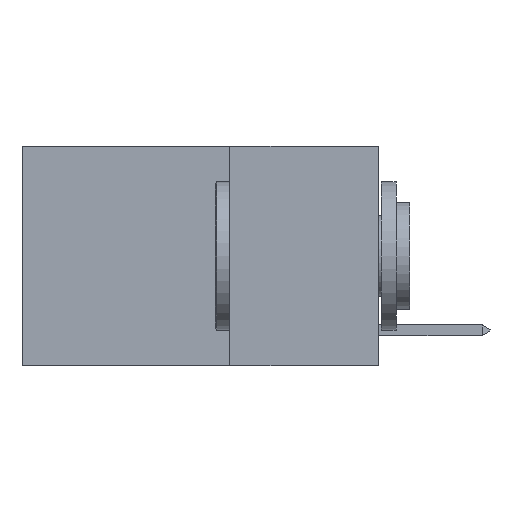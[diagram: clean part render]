
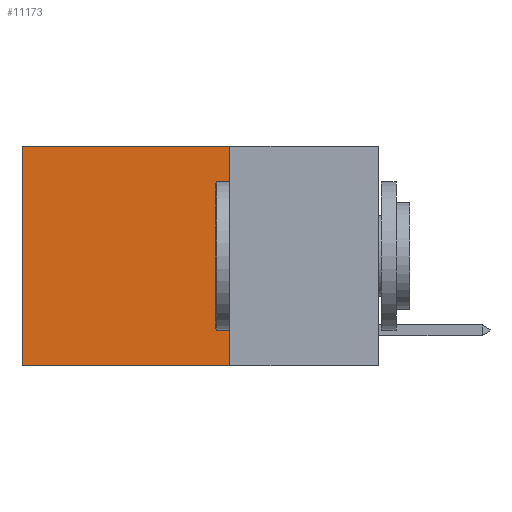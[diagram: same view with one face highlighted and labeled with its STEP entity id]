
A CAD part, left-side view. The second image highlights one B-rep face of the part: STEP entity #11173.
In plain terms, the highlighted planar face has unit normal (-1, 0, 0).
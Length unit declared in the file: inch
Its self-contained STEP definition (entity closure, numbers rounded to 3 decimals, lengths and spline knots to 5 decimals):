
#128 = CARTESIAN_POINT ( 'NONE',  ( 0.2625, 0.25, 0. ) ) ;
#1130 = VERTEX_POINT ( 'NONE', #2008 ) ;
#1347 = CARTESIAN_POINT ( 'NONE',  ( 0.2625, 0.25, 0. ) ) ;
#2008 = CARTESIAN_POINT ( 'NONE',  ( 0.2625, 0.25, -0.37 ) ) ;
#2439 = VERTEX_POINT ( 'NONE', #25533 ) ;
#2777 = LINE ( 'NONE', #7837, #9611 ) ;
#3195 = LINE ( 'NONE', #20239, #3283 ) ;
#3283 = VECTOR ( 'NONE', #17884, 39.37008 ) ;
#4053 = ORIENTED_EDGE ( 'NONE', *, *, #23389, .T. ) ;
#7161 = CARTESIAN_POINT ( 'NONE',  ( 0.2625, 0.25, 0. ) ) ;
#7238 = LINE ( 'NONE', #128, #30230 ) ;
#7837 = CARTESIAN_POINT ( 'NONE',  ( 0.2625, 0.6, 0. ) ) ;
#9611 = VECTOR ( 'NONE', #24683, 39.37008 ) ;
#10201 = EDGE_CURVE ( 'NONE', #1130, #24679, #3195, .T. ) ;
#11173 = ADVANCED_FACE ( 'NONE', ( #16488 ), #25752, .F. ) ;
#11301 = DIRECTION ( 'NONE',  ( 0., 1., 0. ) ) ;
#11524 = DIRECTION ( 'NONE',  ( 0., 0., -1. ) ) ;
#12385 = EDGE_LOOP ( 'NONE', ( #18802, #28247, #30572, #4053 ) ) ;
#13137 = CARTESIAN_POINT ( 'NONE',  ( 0.2625, 0.25, 0. ) ) ;
#13967 = DIRECTION ( 'NONE',  ( 1., 0., 0. ) ) ;
#16456 = AXIS2_PLACEMENT_3D ( 'NONE', #7161, #13967, #23706 ) ;
#16488 = FACE_OUTER_BOUND ( 'NONE', #12385, .T. ) ;
#16555 = VECTOR ( 'NONE', #11301, 39.37008 ) ;
#17884 = DIRECTION ( 'NONE',  ( 0., 1., 0. ) ) ;
#17928 = LINE ( 'NONE', #1347, #16555 ) ;
#18802 = ORIENTED_EDGE ( 'NONE', *, *, #25577, .T. ) ;
#19307 = EDGE_CURVE ( 'NONE', #24839, #1130, #7238, .T. ) ;
#19828 = CARTESIAN_POINT ( 'NONE',  ( 0.2625, 0.6, -0.37 ) ) ;
#20239 = CARTESIAN_POINT ( 'NONE',  ( 0.2625, 0.25, -0.37 ) ) ;
#23389 = EDGE_CURVE ( 'NONE', #24839, #2439, #17928, .T. ) ;
#23706 = DIRECTION ( 'NONE',  ( 0., 0., -1. ) ) ;
#24679 = VERTEX_POINT ( 'NONE', #19828 ) ;
#24683 = DIRECTION ( 'NONE',  ( 0., 0., -1. ) ) ;
#24839 = VERTEX_POINT ( 'NONE', #13137 ) ;
#25533 = CARTESIAN_POINT ( 'NONE',  ( 0.2625, 0.6, 0. ) ) ;
#25577 = EDGE_CURVE ( 'NONE', #2439, #24679, #2777, .T. ) ;
#25752 = PLANE ( 'NONE',  #16456 ) ;
#28247 = ORIENTED_EDGE ( 'NONE', *, *, #10201, .F. ) ;
#30230 = VECTOR ( 'NONE', #11524, 39.37008 ) ;
#30572 = ORIENTED_EDGE ( 'NONE', *, *, #19307, .F. ) ;
